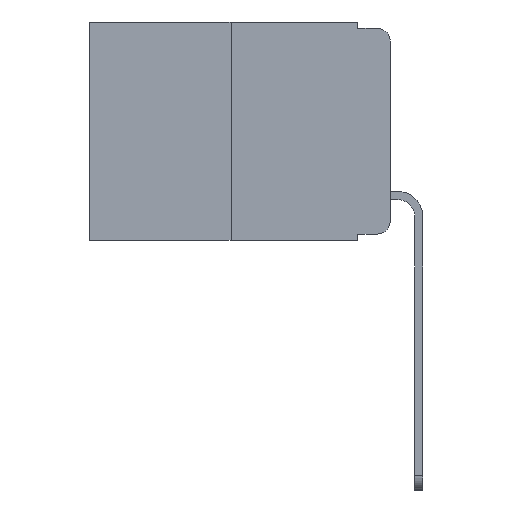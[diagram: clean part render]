
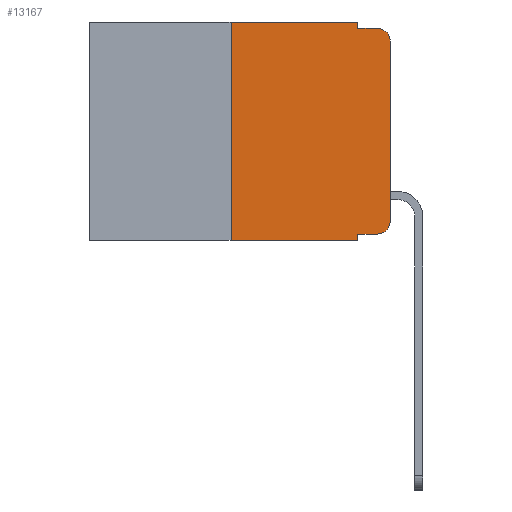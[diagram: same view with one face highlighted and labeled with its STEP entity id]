
A CAD part, left-side view. The second image highlights one B-rep face of the part: STEP entity #13167.
In plain terms, the highlighted planar face has unit normal (-1, 0, 0).
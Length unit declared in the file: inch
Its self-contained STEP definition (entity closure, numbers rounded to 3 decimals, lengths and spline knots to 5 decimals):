
#106 = DIRECTION ( 'NONE',  ( -1., 0., 0. ) ) ;
#166 = CARTESIAN_POINT ( 'NONE',  ( 0., 0.051, 0. ) ) ;
#804 = EDGE_CURVE ( 'NONE', #18231, #6328, #4977, .T. ) ;
#833 = ORIENTED_EDGE ( 'NONE', *, *, #16239, .T. ) ;
#1024 = ORIENTED_EDGE ( 'NONE', *, *, #11325, .F. ) ;
#1038 = ORIENTED_EDGE ( 'NONE', *, *, #18711, .T. ) ;
#1246 = DIRECTION ( 'NONE',  ( 1., 0., 0. ) ) ;
#1265 = DIRECTION ( 'NONE',  ( 0., 0., -1. ) ) ;
#1346 = VECTOR ( 'NONE', #11747, 39.37008 ) ;
#1434 = CARTESIAN_POINT ( 'NONE',  ( 0., 0.051, 0. ) ) ;
#1839 = ORIENTED_EDGE ( 'NONE', *, *, #804, .T. ) ;
#2197 = ORIENTED_EDGE ( 'NONE', *, *, #10310, .F. ) ;
#2425 = ORIENTED_EDGE ( 'NONE', *, *, #12309, .F. ) ;
#2669 = VERTEX_POINT ( 'NONE', #13301 ) ;
#2960 = ORIENTED_EDGE ( 'NONE', *, *, #4444, .T. ) ;
#3209 = LINE ( 'NONE', #8884, #10537 ) ;
#3607 = VECTOR ( 'NONE', #12363, 39.37008 ) ;
#3730 = CARTESIAN_POINT ( 'NONE',  ( 0., 0.25, 0. ) ) ;
#4370 = CARTESIAN_POINT ( 'NONE',  ( 0., 0.051, -0.01 ) ) ;
#4397 = ORIENTED_EDGE ( 'NONE', *, *, #6429, .T. ) ;
#4442 = ORIENTED_EDGE ( 'NONE', *, *, #7360, .F. ) ;
#4444 = EDGE_CURVE ( 'NONE', #6328, #8576, #3209, .T. ) ;
#4448 = AXIS2_PLACEMENT_3D ( 'NONE', #18844, #10250, #1265 ) ;
#4977 = CIRCLE ( 'NONE', #12476, 0.02 ) ;
#5054 = EDGE_LOOP ( 'NONE', ( #2960, #4397, #4442, #2197, #9015, #1024, #1038, #2425, #833, #1839 ) ) ;
#5666 = VERTEX_POINT ( 'NONE', #1434 ) ;
#5967 = LINE ( 'NONE', #10224, #1346 ) ;
#6328 = VERTEX_POINT ( 'NONE', #18668 ) ;
#6429 = EDGE_CURVE ( 'NONE', #8576, #10199, #16639, .T. ) ;
#6610 = VECTOR ( 'NONE', #14009, 39.37008 ) ;
#7239 = CARTESIAN_POINT ( 'NONE',  ( 0., 0.473, 0. ) ) ;
#7360 = EDGE_CURVE ( 'NONE', #19145, #10199, #12946, .T. ) ;
#7766 = VECTOR ( 'NONE', #10803, 39.37008 ) ;
#8213 = LINE ( 'NONE', #9349, #7766 ) ;
#8231 = CARTESIAN_POINT ( 'NONE',  ( 0., 0.02, -0.313 ) ) ;
#8576 = VERTEX_POINT ( 'NONE', #14182 ) ;
#8884 = CARTESIAN_POINT ( 'NONE',  ( 0., 0., 0. ) ) ;
#9015 = ORIENTED_EDGE ( 'NONE', *, *, #16057, .F. ) ;
#9349 = CARTESIAN_POINT ( 'NONE',  ( 0., 0.051, 0. ) ) ;
#9649 = CARTESIAN_POINT ( 'NONE',  ( 0., 0.051, -0.343 ) ) ;
#9829 = DIRECTION ( 'NONE',  ( 0., -1., 0. ) ) ;
#10199 = VERTEX_POINT ( 'NONE', #13393 ) ;
#10224 = CARTESIAN_POINT ( 'NONE',  ( 0., 0.051, -0.333 ) ) ;
#10230 = PLANE ( 'NONE',  #11151 ) ;
#10250 = DIRECTION ( 'NONE',  ( -1., 0., 0. ) ) ;
#10310 = EDGE_CURVE ( 'NONE', #5666, #19145, #8213, .T. ) ;
#10435 = CARTESIAN_POINT ( 'NONE',  ( 0., 0.473, -0.343 ) ) ;
#10537 = VECTOR ( 'NONE', #11888, 39.37008 ) ;
#10803 = DIRECTION ( 'NONE',  ( 0., 0., -1. ) ) ;
#11151 = AXIS2_PLACEMENT_3D ( 'NONE', #7239, #1246, #11758 ) ;
#11325 = EDGE_CURVE ( 'NONE', #19103, #2669, #11421, .T. ) ;
#11407 = LINE ( 'NONE', #166, #3607 ) ;
#11421 = LINE ( 'NONE', #3730, #6610 ) ;
#11678 = VECTOR ( 'NONE', #9829, 39.37008 ) ;
#11747 = DIRECTION ( 'NONE',  ( 0., -1., 0. ) ) ;
#11758 = DIRECTION ( 'NONE',  ( 0., 0., -1. ) ) ;
#11888 = DIRECTION ( 'NONE',  ( 0., 0., 1. ) ) ;
#12309 = EDGE_CURVE ( 'NONE', #16234, #15955, #11407, .T. ) ;
#12363 = DIRECTION ( 'NONE',  ( 0., 0., -1. ) ) ;
#12476 = AXIS2_PLACEMENT_3D ( 'NONE', #8231, #106, #17032 ) ;
#12946 = LINE ( 'NONE', #4370, #13410 ) ;
#12948 = CARTESIAN_POINT ( 'NONE',  ( 0., 0.051, -0.01 ) ) ;
#13167 = ADVANCED_FACE ( 'NONE', ( #16821 ), #10230, .F. ) ;
#13301 = CARTESIAN_POINT ( 'NONE',  ( 0., 0.25, 0. ) ) ;
#13393 = CARTESIAN_POINT ( 'NONE',  ( 0., 0.02, -0.01 ) ) ;
#13410 = VECTOR ( 'NONE', #16110, 39.37008 ) ;
#13931 = LINE ( 'NONE', #10435, #17270 ) ;
#14009 = DIRECTION ( 'NONE',  ( 0., 0., 1. ) ) ;
#14182 = CARTESIAN_POINT ( 'NONE',  ( 0., 0., -0.03 ) ) ;
#15774 = CARTESIAN_POINT ( 'NONE',  ( 0., 0.25, -0.343 ) ) ;
#15955 = VERTEX_POINT ( 'NONE', #9649 ) ;
#16044 = LINE ( 'NONE', #18475, #11678 ) ;
#16057 = EDGE_CURVE ( 'NONE', #2669, #5666, #16044, .T. ) ;
#16110 = DIRECTION ( 'NONE',  ( 0., -1., 0. ) ) ;
#16112 = CARTESIAN_POINT ( 'NONE',  ( 0., 0.051, -0.333 ) ) ;
#16234 = VERTEX_POINT ( 'NONE', #16112 ) ;
#16239 = EDGE_CURVE ( 'NONE', #16234, #18231, #5967, .T. ) ;
#16639 = CIRCLE ( 'NONE', #4448, 0.02 ) ;
#16821 = FACE_OUTER_BOUND ( 'NONE', #5054, .T. ) ;
#17032 = DIRECTION ( 'NONE',  ( 0., 0., -1. ) ) ;
#17270 = VECTOR ( 'NONE', #17711, 39.37008 ) ;
#17711 = DIRECTION ( 'NONE',  ( 0., -1., 0. ) ) ;
#18188 = CARTESIAN_POINT ( 'NONE',  ( 0., 0.02, -0.333 ) ) ;
#18231 = VERTEX_POINT ( 'NONE', #18188 ) ;
#18475 = CARTESIAN_POINT ( 'NONE',  ( 0., 0.473, 0. ) ) ;
#18668 = CARTESIAN_POINT ( 'NONE',  ( 0., 0., -0.313 ) ) ;
#18711 = EDGE_CURVE ( 'NONE', #19103, #15955, #13931, .T. ) ;
#18844 = CARTESIAN_POINT ( 'NONE',  ( 0., 0.02, -0.03 ) ) ;
#19103 = VERTEX_POINT ( 'NONE', #15774 ) ;
#19145 = VERTEX_POINT ( 'NONE', #12948 ) ;
